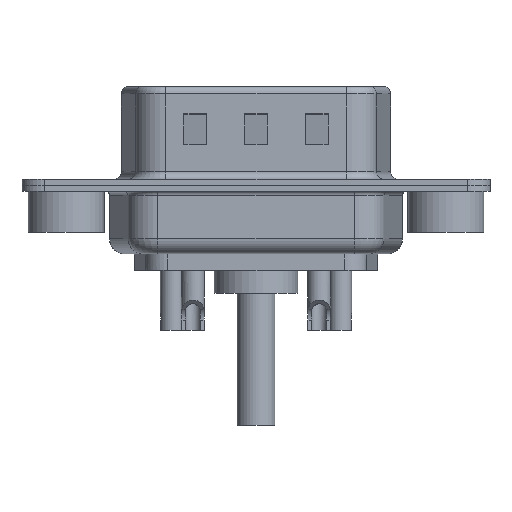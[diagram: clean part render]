
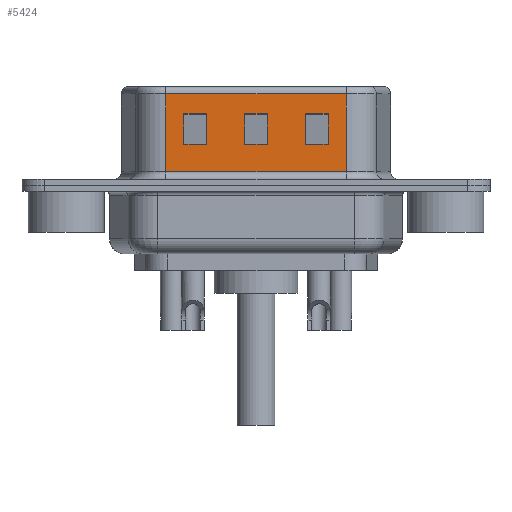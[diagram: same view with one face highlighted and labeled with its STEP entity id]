
A CAD part, front view. The second image highlights one B-rep face of the part: STEP entity #5424.
In plain terms, the highlighted planar face has unit normal (0, -1, 0).
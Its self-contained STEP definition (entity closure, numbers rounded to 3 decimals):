
#255 = LINE ( 'NONE', #10671, #3434 ) ;
#405 = LINE ( 'NONE', #3446, #14120 ) ;
#535 = EDGE_LOOP ( 'NONE', ( #8556, #1179, #12779, #3314 ) ) ;
#677 = LINE ( 'NONE', #6501, #11027 ) ;
#865 = ORIENTED_EDGE ( 'NONE', *, *, #13815, .T. ) ;
#968 = CARTESIAN_POINT ( 'NONE',  ( 11.75, -4.58, 4.705 ) ) ;
#1105 = DIRECTION ( 'NONE',  ( 0., 0., -1. ) ) ;
#1126 = CARTESIAN_POINT ( 'NONE',  ( 18.45, -4.58, 0.9 ) ) ;
#1179 = ORIENTED_EDGE ( 'NONE', *, *, #6031, .T. ) ;
#1248 = VECTOR ( 'NONE', #16867, 1000. ) ;
#1543 = CARTESIAN_POINT ( 'NONE',  ( 18.45, -4.58, 6.02 ) ) ;
#1769 = EDGE_CURVE ( 'NONE', #11289, #4009, #12052, .T. ) ;
#1871 = CARTESIAN_POINT ( 'NONE',  ( 6.55, -4.58, 0.9 ) ) ;
#1900 = EDGE_CURVE ( 'NONE', #11767, #4739, #7254, .T. ) ;
#2190 = EDGE_CURVE ( 'NONE', #14957, #8523, #255, .T. ) ;
#2348 = VECTOR ( 'NONE', #15624, 1000. ) ;
#2374 = DIRECTION ( 'NONE',  ( 0., 0., 1. ) ) ;
#2413 = VERTEX_POINT ( 'NONE', #15322 ) ;
#2457 = VERTEX_POINT ( 'NONE', #3960 ) ;
#2520 = EDGE_CURVE ( 'NONE', #14957, #12885, #9961, .T. ) ;
#2524 = CARTESIAN_POINT ( 'NONE',  ( 7.75, -4.58, 2.705 ) ) ;
#2698 = CARTESIAN_POINT ( 'NONE',  ( 9.25, -4.58, 2.705 ) ) ;
#2779 = DIRECTION ( 'NONE',  ( 0., 1., 0. ) ) ;
#2807 = VECTOR ( 'NONE', #3908, 1000. ) ;
#2818 = VECTOR ( 'NONE', #15775, 1000. ) ;
#3220 = LINE ( 'NONE', #15320, #9555 ) ;
#3314 = ORIENTED_EDGE ( 'NONE', *, *, #16301, .T. ) ;
#3399 = CARTESIAN_POINT ( 'NONE',  ( 22.45, -4.58, 2.705 ) ) ;
#3421 = LINE ( 'NONE', #7384, #7872 ) ;
#3432 = EDGE_LOOP ( 'NONE', ( #9806, #8576, #8321, #3941 ) ) ;
#3434 = VECTOR ( 'NONE', #13583, 1000. ) ;
#3446 = CARTESIAN_POINT ( 'NONE',  ( 6.55, -4.58, 6.52 ) ) ;
#3720 = EDGE_CURVE ( 'NONE', #5940, #7583, #3421, .T. ) ;
#3757 = DIRECTION ( 'NONE',  ( 1., 0., 0. ) ) ;
#3832 = LINE ( 'NONE', #3399, #10153 ) ;
#3908 = DIRECTION ( 'NONE',  ( 0., 0., -1. ) ) ;
#3941 = ORIENTED_EDGE ( 'NONE', *, *, #8615, .T. ) ;
#3960 = CARTESIAN_POINT ( 'NONE',  ( 7.75, -4.58, 4.705 ) ) ;
#4009 = VERTEX_POINT ( 'NONE', #4357 ) ;
#4357 = CARTESIAN_POINT ( 'NONE',  ( 17.25, -4.58, 2.705 ) ) ;
#4394 = LINE ( 'NONE', #10438, #10697 ) ;
#4454 = VECTOR ( 'NONE', #13157, 1000. ) ;
#4511 = ORIENTED_EDGE ( 'NONE', *, *, #13047, .T. ) ;
#4700 = DIRECTION ( 'NONE',  ( 0., 0., 1. ) ) ;
#4739 = VERTEX_POINT ( 'NONE', #11452 ) ;
#4858 = LINE ( 'NONE', #16814, #1248 ) ;
#4882 = EDGE_LOOP ( 'NONE', ( #6379, #4511, #14095, #9515 ) ) ;
#5099 = CARTESIAN_POINT ( 'NONE',  ( 7.75, -4.58, 6.52 ) ) ;
#5255 = CARTESIAN_POINT ( 'NONE',  ( 14.45, -4.58, 2.705 ) ) ;
#5424 = ADVANCED_FACE ( 'NONE', ( #8033, #15719, #14908, #14513 ), #14585, .F. ) ;
#5777 = CARTESIAN_POINT ( 'NONE',  ( 18.45, -4.58, 0.9 ) ) ;
#5940 = VERTEX_POINT ( 'NONE', #968 ) ;
#5974 = EDGE_CURVE ( 'NONE', #4739, #11289, #4858, .T. ) ;
#6031 = EDGE_CURVE ( 'NONE', #9713, #9668, #11562, .T. ) ;
#6379 = ORIENTED_EDGE ( 'NONE', *, *, #1769, .T. ) ;
#6430 = CARTESIAN_POINT ( 'NONE',  ( 14.45, -4.58, 4.705 ) ) ;
#6447 = VERTEX_POINT ( 'NONE', #1871 ) ;
#6501 = CARTESIAN_POINT ( 'NONE',  ( 9.25, -4.58, 6.52 ) ) ;
#6924 = CARTESIAN_POINT ( 'NONE',  ( 13.25, -4.58, 4.705 ) ) ;
#7106 = VERTEX_POINT ( 'NONE', #15037 ) ;
#7254 = LINE ( 'NONE', #11577, #10411 ) ;
#7384 = CARTESIAN_POINT ( 'NONE',  ( 18.45, -4.58, 4.705 ) ) ;
#7541 = LINE ( 'NONE', #5099, #17040 ) ;
#7583 = VERTEX_POINT ( 'NONE', #6924 ) ;
#7587 = DIRECTION ( 'NONE',  ( -1., 0., 0. ) ) ;
#7843 = CARTESIAN_POINT ( 'NONE',  ( 18.45, -4.58, 6.52 ) ) ;
#7872 = VECTOR ( 'NONE', #15926, 1000. ) ;
#8033 = FACE_BOUND ( 'NONE', #535, .T. ) ;
#8321 = ORIENTED_EDGE ( 'NONE', *, *, #12257, .T. ) ;
#8373 = CARTESIAN_POINT ( 'NONE',  ( 17.25, -4.58, 4.705 ) ) ;
#8523 = VERTEX_POINT ( 'NONE', #14045 ) ;
#8556 = ORIENTED_EDGE ( 'NONE', *, *, #15514, .T. ) ;
#8576 = ORIENTED_EDGE ( 'NONE', *, *, #15376, .T. ) ;
#8615 = EDGE_CURVE ( 'NONE', #7106, #5940, #4394, .T. ) ;
#8636 = EDGE_CURVE ( 'NONE', #9668, #2457, #7541, .T. ) ;
#9515 = ORIENTED_EDGE ( 'NONE', *, *, #5974, .T. ) ;
#9555 = VECTOR ( 'NONE', #7587, 1000. ) ;
#9668 = VERTEX_POINT ( 'NONE', #2524 ) ;
#9713 = VERTEX_POINT ( 'NONE', #2698 ) ;
#9806 = ORIENTED_EDGE ( 'NONE', *, *, #3720, .T. ) ;
#9961 = LINE ( 'NONE', #7843, #2807 ) ;
#10153 = VECTOR ( 'NONE', #11448, 1000. ) ;
#10411 = VECTOR ( 'NONE', #4700, 1000. ) ;
#10438 = CARTESIAN_POINT ( 'NONE',  ( 11.75, -4.58, 6.52 ) ) ;
#10671 = CARTESIAN_POINT ( 'NONE',  ( 18.45, -4.58, 6.02 ) ) ;
#10697 = VECTOR ( 'NONE', #2374, 1000. ) ;
#11027 = VECTOR ( 'NONE', #1105, 1000. ) ;
#11289 = VERTEX_POINT ( 'NONE', #8373 ) ;
#11448 = DIRECTION ( 'NONE',  ( -1., 0., 0. ) ) ;
#11452 = CARTESIAN_POINT ( 'NONE',  ( 15.75, -4.58, 4.705 ) ) ;
#11562 = LINE ( 'NONE', #5255, #4454 ) ;
#11577 = CARTESIAN_POINT ( 'NONE',  ( 15.75, -4.58, 6.52 ) ) ;
#11767 = VERTEX_POINT ( 'NONE', #11913 ) ;
#11913 = CARTESIAN_POINT ( 'NONE',  ( 15.75, -4.58, 2.705 ) ) ;
#12035 = CARTESIAN_POINT ( 'NONE',  ( 13.25, -4.58, 2.705 ) ) ;
#12052 = LINE ( 'NONE', #16589, #14974 ) ;
#12084 = EDGE_LOOP ( 'NONE', ( #13881, #13816, #865, #14508 ) ) ;
#12142 = DIRECTION ( 'NONE',  ( 0., 0., 1. ) ) ;
#12257 = EDGE_CURVE ( 'NONE', #12704, #7106, #3220, .T. ) ;
#12704 = VERTEX_POINT ( 'NONE', #12035 ) ;
#12779 = ORIENTED_EDGE ( 'NONE', *, *, #8636, .T. ) ;
#12805 = VECTOR ( 'NONE', #3757, 1000. ) ;
#12885 = VERTEX_POINT ( 'NONE', #5777 ) ;
#13047 = EDGE_CURVE ( 'NONE', #4009, #11767, #3832, .T. ) ;
#13157 = DIRECTION ( 'NONE',  ( -1., 0., 0. ) ) ;
#13583 = DIRECTION ( 'NONE',  ( -1., 0., 0. ) ) ;
#13815 = EDGE_CURVE ( 'NONE', #8523, #6447, #405, .T. ) ;
#13816 = ORIENTED_EDGE ( 'NONE', *, *, #2190, .T. ) ;
#13881 = ORIENTED_EDGE ( 'NONE', *, *, #2520, .F. ) ;
#13940 = EDGE_CURVE ( 'NONE', #6447, #12885, #16311, .T. ) ;
#14045 = CARTESIAN_POINT ( 'NONE',  ( 6.55, -4.58, 6.02 ) ) ;
#14095 = ORIENTED_EDGE ( 'NONE', *, *, #1900, .T. ) ;
#14120 = VECTOR ( 'NONE', #15264, 1000. ) ;
#14262 = DIRECTION ( 'NONE',  ( 0., 0., 1. ) ) ;
#14483 = CARTESIAN_POINT ( 'NONE',  ( 13.25, -4.58, 6.52 ) ) ;
#14508 = ORIENTED_EDGE ( 'NONE', *, *, #13940, .T. ) ;
#14513 = FACE_OUTER_BOUND ( 'NONE', #12084, .T. ) ;
#14585 = PLANE ( 'NONE',  #16131 ) ;
#14908 = FACE_BOUND ( 'NONE', #3432, .T. ) ;
#14957 = VERTEX_POINT ( 'NONE', #1543 ) ;
#14974 = VECTOR ( 'NONE', #16389, 1000. ) ;
#15037 = CARTESIAN_POINT ( 'NONE',  ( 11.75, -4.58, 2.705 ) ) ;
#15264 = DIRECTION ( 'NONE',  ( 0., 0., -1. ) ) ;
#15320 = CARTESIAN_POINT ( 'NONE',  ( 18.45, -4.58, 2.705 ) ) ;
#15322 = CARTESIAN_POINT ( 'NONE',  ( 9.25, -4.58, 4.705 ) ) ;
#15376 = EDGE_CURVE ( 'NONE', #7583, #12704, #16366, .T. ) ;
#15514 = EDGE_CURVE ( 'NONE', #2413, #9713, #677, .T. ) ;
#15624 = DIRECTION ( 'NONE',  ( 1., 0., 0. ) ) ;
#15719 = FACE_BOUND ( 'NONE', #4882, .T. ) ;
#15775 = DIRECTION ( 'NONE',  ( 0., 0., -1. ) ) ;
#15872 = CARTESIAN_POINT ( 'NONE',  ( 18.45, -4.58, 6.52 ) ) ;
#15926 = DIRECTION ( 'NONE',  ( 1., 0., 0. ) ) ;
#16131 = AXIS2_PLACEMENT_3D ( 'NONE', #15872, #2779, #12142 ) ;
#16138 = LINE ( 'NONE', #6430, #12805 ) ;
#16301 = EDGE_CURVE ( 'NONE', #2457, #2413, #16138, .T. ) ;
#16311 = LINE ( 'NONE', #1126, #2348 ) ;
#16366 = LINE ( 'NONE', #14483, #2818 ) ;
#16389 = DIRECTION ( 'NONE',  ( 0., 0., -1. ) ) ;
#16589 = CARTESIAN_POINT ( 'NONE',  ( 17.25, -4.58, 6.52 ) ) ;
#16814 = CARTESIAN_POINT ( 'NONE',  ( 22.45, -4.58, 4.705 ) ) ;
#16867 = DIRECTION ( 'NONE',  ( 1., 0., 0. ) ) ;
#17040 = VECTOR ( 'NONE', #14262, 1000. ) ;
